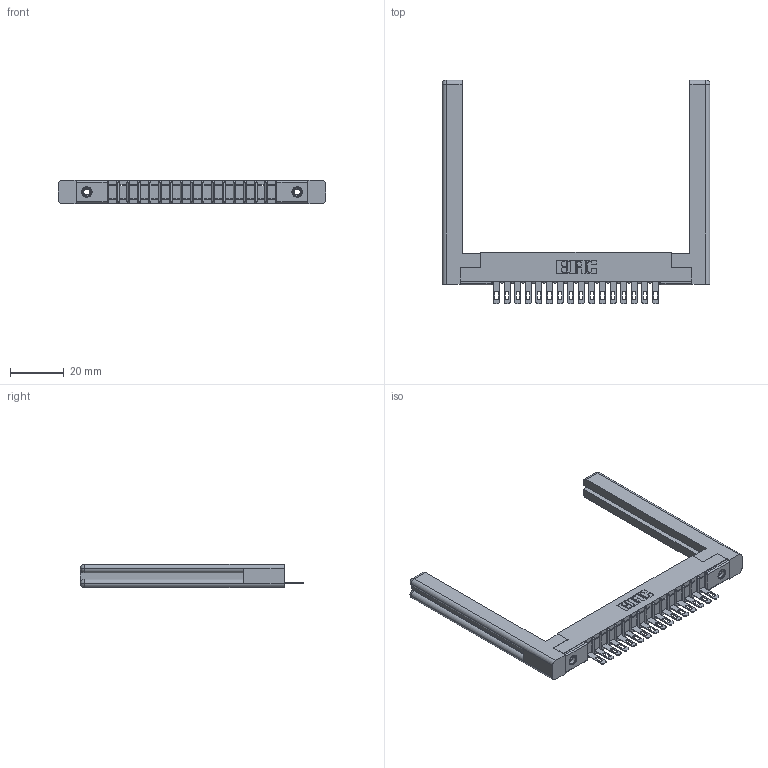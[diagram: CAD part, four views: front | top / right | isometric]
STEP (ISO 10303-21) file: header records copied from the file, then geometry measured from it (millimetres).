
FILE_DESCRIPTION (( 'STEP AP203' ), '1' );
FILE_NAME ('357-016-405-158.STEP', '2020-09-30T18:32:13', ( '' ), ( '' ), 'SwSTEP 2.0', 'SolidWorks 2020', '' );
FILE_SCHEMA (( 'CONFIG_CONTROL_DESIGN' ));
Length unit declared in the file: inch
Products named in the file (5): 357-016-405-158; 307-290-001_505; 307 Part_.156 Dia Mounting Holes; 307-220-058; 345-250-001_345-250-001-102
Assembly tree (21 placements, depth 2):
  357-016-405-158
    307 Part_.156 Dia Mounting Holes
    307-290-001_505  x16
    307-220-058  x2
    345-250-001_345-250-001-102  x2
Bounding box: 100.03 x 83.49 x 8.71 mm (x, y, z)
Volume: 14069.4 mm3; surface area: 15085.9 mm2
Topology: 21 solids, 21 shells, 1173 faces, 3269 edges, 2098 vertices
Faces by surface type: plane 730, cylinder 385, sphere 34, torus 12, cone 12
Entity records: 19529 total; most frequent: CARTESIAN_POINT 3287, ORIENTED_EDGE 3212, DIRECTION 3174, EDGE_CURVE 1606, LINE 1216, VECTOR 1216, VERTEX_POINT 1038, AXIS2_PLACEMENT_3D 979
